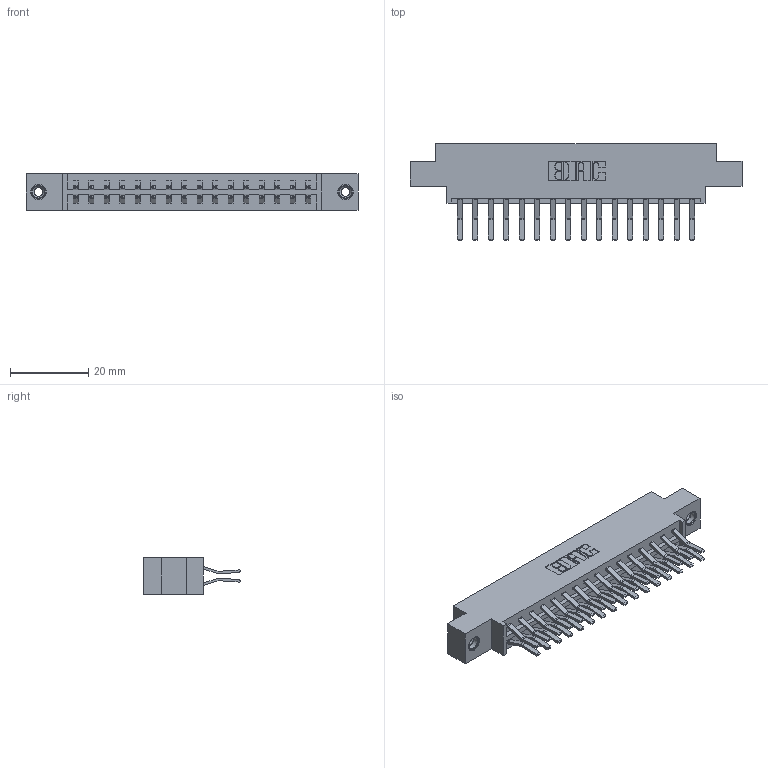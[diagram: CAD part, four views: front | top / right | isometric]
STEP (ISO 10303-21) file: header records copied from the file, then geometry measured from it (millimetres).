
FILE_DESCRIPTION (( 'STEP AP203' ), '1' );
FILE_NAME ('833-032-560-808.STEP', '2020-06-02T19:36:26', ( '' ), ( '' ), 'SwSTEP 2.0', 'SolidWorks 2020', '' );
FILE_SCHEMA (( 'CONFIG_CONTROL_DESIGN' ));
Length unit declared in the file: inch
Products named in the file (4): 345-292-001_560 Tail; 345-250-001_345-250-003-102; 833 Part_Offset - .156 Dia - TI; 833-032-560-808
Assembly tree (35 placements, depth 2):
  833-032-560-808
    833 Part_Offset - .156 Dia - TI
    345-292-001_560 Tail  x32
    345-250-001_345-250-003-102  x2
Bounding box: 84.94 x 24.78 x 9.4 mm (x, y, z)
Volume: 8403.9 mm3; surface area: 10497.1 mm2
Topology: 35 solids, 35 shells, 1906 faces, 5611 edges, 3690 vertices
Faces by surface type: plane 1258, cylinder 632, cone 12, torus 4
Entity records: 15062 total; most frequent: CARTESIAN_POINT 2513, ORIENTED_EDGE 2442, DIRECTION 2227, EDGE_CURVE 1221, VECTOR 1069, LINE 1069, VERTEX_POINT 808, AXIS2_PLACEMENT_3D 579
